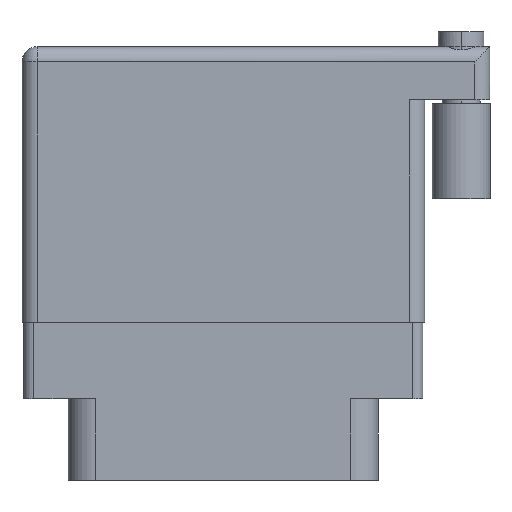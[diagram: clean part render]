
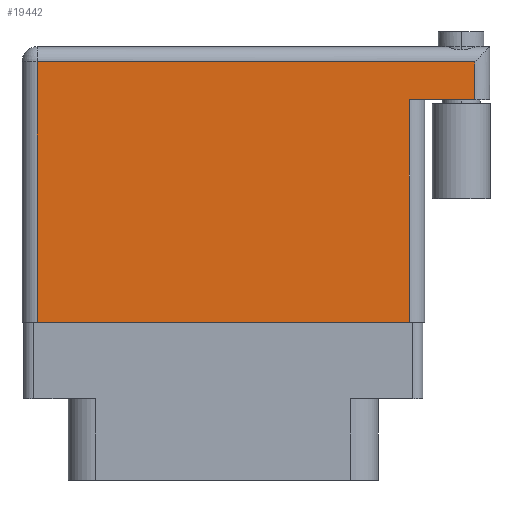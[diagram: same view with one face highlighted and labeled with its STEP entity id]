
A CAD part, front view. The second image highlights one B-rep face of the part: STEP entity #19442.
In plain terms, the highlighted face is planar.
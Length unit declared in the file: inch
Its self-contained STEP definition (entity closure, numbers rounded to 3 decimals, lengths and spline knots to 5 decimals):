
#1184 = EDGE_CURVE ( 'NONE', #7792, #15549, #7777, .T. ) ;
#1628 = VERTEX_POINT ( 'NONE', #20401 ) ;
#1820 = CARTESIAN_POINT ( 'NONE',  ( 1.489, 0.731, 0. ) ) ;
#1837 = VERTEX_POINT ( 'NONE', #17752 ) ;
#1845 = VECTOR ( 'NONE', #8503, 39.37008 ) ;
#3688 = FACE_OUTER_BOUND ( 'NONE', #17200, .T. ) ;
#4248 = EDGE_CURVE ( 'NONE', #1628, #14760, #14377, .T. ) ;
#4267 = CARTESIAN_POINT ( 'NONE',  ( 0., 0., 0. ) ) ;
#6500 = CARTESIAN_POINT ( 'NONE',  ( 1.489, 0.906, 0. ) ) ;
#6751 = DIRECTION ( 'NONE',  ( 0., 1., 0. ) ) ;
#7302 = ORIENTED_EDGE ( 'NONE', *, *, #19686, .T. ) ;
#7777 = LINE ( 'NONE', #6500, #19984 ) ;
#7792 = VERTEX_POINT ( 'NONE', #1820 ) ;
#8395 = DIRECTION ( 'NONE',  ( -1., 0., 0. ) ) ;
#8413 = DIRECTION ( 'NONE',  ( 0., 1., 0. ) ) ;
#8503 = DIRECTION ( 'NONE',  ( -1., 0., 0. ) ) ;
#9054 = VECTOR ( 'NONE', #10506, 39.37008 ) ;
#10265 = ORIENTED_EDGE ( 'NONE', *, *, #21764, .T. ) ;
#10506 = DIRECTION ( 'NONE',  ( 0., -1., 0. ) ) ;
#11205 = ORIENTED_EDGE ( 'NONE', *, *, #4248, .T. ) ;
#12338 = VECTOR ( 'NONE', #6751, 39.37008 ) ;
#12705 = CARTESIAN_POINT ( 'NONE',  ( 0., 0.856, 0. ) ) ;
#12856 = CARTESIAN_POINT ( 'NONE',  ( 1.275, 0.731, 0. ) ) ;
#13536 = ORIENTED_EDGE ( 'NONE', *, *, #1184, .T. ) ;
#14008 = LINE ( 'NONE', #20412, #23637 ) ;
#14377 = LINE ( 'NONE', #4267, #19546 ) ;
#14760 = VERTEX_POINT ( 'NONE', #22705 ) ;
#14897 = ORIENTED_EDGE ( 'NONE', *, *, #22539, .T. ) ;
#15549 = VERTEX_POINT ( 'NONE', #23481 ) ;
#15895 = DIRECTION ( 'NONE',  ( -1., 0., 0. ) ) ;
#16440 = DIRECTION ( 'NONE',  ( 1., 0., 0. ) ) ;
#16577 = CARTESIAN_POINT ( 'NONE',  ( 0.05, 0., 0. ) ) ;
#17200 = EDGE_LOOP ( 'NONE', ( #11205, #14897, #24252, #13536, #10265, #7302 ) ) ;
#17752 = CARTESIAN_POINT ( 'NONE',  ( 1.275, 0.731, 0. ) ) ;
#18192 = VERTEX_POINT ( 'NONE', #21336 ) ;
#18516 = EDGE_CURVE ( 'NONE', #7792, #1837, #14008, .T. ) ;
#19442 = ADVANCED_FACE ( 'NONE', ( #3688 ), #23793, .F. ) ;
#19546 = VECTOR ( 'NONE', #16440, 39.37008 ) ;
#19686 = EDGE_CURVE ( 'NONE', #18192, #1628, #25382, .T. ) ;
#19984 = VECTOR ( 'NONE', #8413, 39.37008 ) ;
#20401 = CARTESIAN_POINT ( 'NONE',  ( 0.05, 0., 0. ) ) ;
#20412 = CARTESIAN_POINT ( 'NONE',  ( 1.539, 0.731, 0. ) ) ;
#20719 = LINE ( 'NONE', #12705, #1845 ) ;
#21336 = CARTESIAN_POINT ( 'NONE',  ( 0.05, 0.856, 0. ) ) ;
#21764 = EDGE_CURVE ( 'NONE', #15549, #18192, #20719, .T. ) ;
#21829 = CARTESIAN_POINT ( 'NONE',  ( 0., 0.906, 0. ) ) ;
#22539 = EDGE_CURVE ( 'NONE', #14760, #1837, #24532, .T. ) ;
#22705 = CARTESIAN_POINT ( 'NONE',  ( 1.275, 0., 0. ) ) ;
#23481 = CARTESIAN_POINT ( 'NONE',  ( 1.489, 0.856, 0. ) ) ;
#23637 = VECTOR ( 'NONE', #8395, 39.37008 ) ;
#23793 = PLANE ( 'NONE',  #24048 ) ;
#24048 = AXIS2_PLACEMENT_3D ( 'NONE', #21829, #26115, #15895 ) ;
#24252 = ORIENTED_EDGE ( 'NONE', *, *, #18516, .F. ) ;
#24532 = LINE ( 'NONE', #12856, #12338 ) ;
#25382 = LINE ( 'NONE', #16577, #9054 ) ;
#26115 = DIRECTION ( 'NONE',  ( 0., 0., -1. ) ) ;
